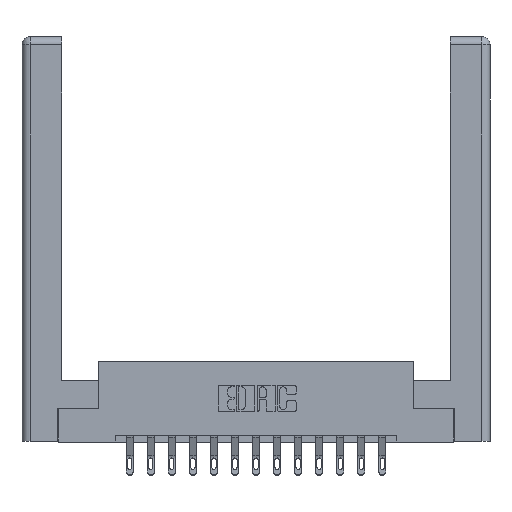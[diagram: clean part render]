
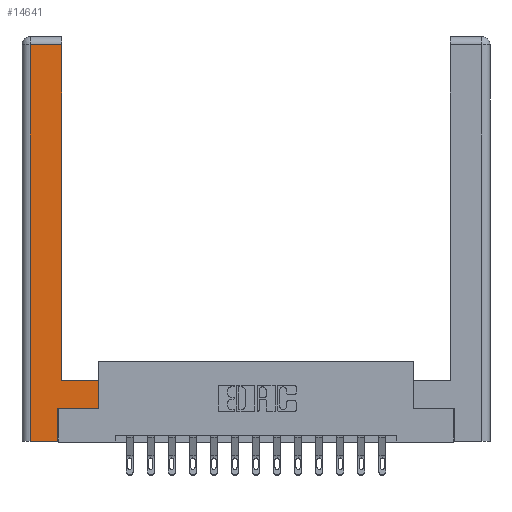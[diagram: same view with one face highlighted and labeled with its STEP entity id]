
A CAD part, top view. The second image highlights one B-rep face of the part: STEP entity #14641.
In plain terms, the highlighted planar face has unit normal (0, 0, 1).
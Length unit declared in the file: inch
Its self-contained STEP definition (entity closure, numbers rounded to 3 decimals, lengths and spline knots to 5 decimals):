
#505 = CARTESIAN_POINT ( 'NONE',  ( 0.565, 0.245, 0. ) ) ;
#565 = VECTOR ( 'NONE', #7714, 39.37008 ) ;
#623 = DIRECTION ( 'NONE',  ( -1., 0., 0. ) ) ;
#813 = VERTEX_POINT ( 'NONE', #505 ) ;
#921 = DIRECTION ( 'NONE',  ( 0., 1., 0. ) ) ;
#1195 = VERTEX_POINT ( 'NONE', #1445 ) ;
#1219 = FACE_OUTER_BOUND ( 'NONE', #9299, .T. ) ;
#1445 = CARTESIAN_POINT ( 'NONE',  ( 0.265, 0., 0. ) ) ;
#1475 = VERTEX_POINT ( 'NONE', #13911 ) ;
#1801 = CARTESIAN_POINT ( 'NONE',  ( 0.0615, 2.94, 0. ) ) ;
#1964 = CARTESIAN_POINT ( 'NONE',  ( 0.0615, 2.94, 0. ) ) ;
#2117 = CARTESIAN_POINT ( 'NONE',  ( 0.0615, 0., 0. ) ) ;
#2124 = CARTESIAN_POINT ( 'NONE',  ( 0.265, 0.245, 0. ) ) ;
#2249 = VECTOR ( 'NONE', #3115, 39.37008 ) ;
#2702 = ORIENTED_EDGE ( 'NONE', *, *, #9964, .T. ) ;
#3115 = DIRECTION ( 'NONE',  ( -1., 0., 0. ) ) ;
#3175 = EDGE_CURVE ( 'NONE', #1195, #6629, #4870, .T. ) ;
#3377 = VERTEX_POINT ( 'NONE', #10694 ) ;
#3609 = PLANE ( 'NONE',  #8350 ) ;
#3668 = LINE ( 'NONE', #12040, #7566 ) ;
#3919 = CARTESIAN_POINT ( 'NONE',  ( 0.565, 0.245, 0. ) ) ;
#4242 = DIRECTION ( 'NONE',  ( 1., 0., 0. ) ) ;
#4404 = ORIENTED_EDGE ( 'NONE', *, *, #7227, .T. ) ;
#4689 = CARTESIAN_POINT ( 'NONE',  ( 0., 0., 0. ) ) ;
#4712 = CARTESIAN_POINT ( 'NONE',  ( 0.0615, 0., 0. ) ) ;
#4793 = CARTESIAN_POINT ( 'NONE',  ( 0.295, 0.45, 0. ) ) ;
#4870 = LINE ( 'NONE', #15410, #565 ) ;
#5075 = VERTEX_POINT ( 'NONE', #1964 ) ;
#5552 = EDGE_CURVE ( 'NONE', #813, #3377, #14548, .T. ) ;
#6075 = VECTOR ( 'NONE', #12247, 39.37008 ) ;
#6571 = LINE ( 'NONE', #1801, #2249 ) ;
#6629 = VERTEX_POINT ( 'NONE', #2124 ) ;
#6631 = DIRECTION ( 'NONE',  ( 1., 0., 0. ) ) ;
#7207 = LINE ( 'NONE', #16402, #10258 ) ;
#7227 = EDGE_CURVE ( 'NONE', #6629, #813, #11699, .T. ) ;
#7566 = VECTOR ( 'NONE', #4242, 39.37008 ) ;
#7714 = DIRECTION ( 'NONE',  ( 0., 1., 0. ) ) ;
#8350 = AXIS2_PLACEMENT_3D ( 'NONE', #4689, #12789, #12743 ) ;
#8803 = ORIENTED_EDGE ( 'NONE', *, *, #13576, .T. ) ;
#9165 = EDGE_CURVE ( 'NONE', #1475, #14554, #7207, .T. ) ;
#9299 = EDGE_LOOP ( 'NONE', ( #14839, #2702, #14176, #10790, #10828, #4404, #13908, #8803 ) ) ;
#9964 = EDGE_CURVE ( 'NONE', #14554, #5075, #6571, .T. ) ;
#10258 = VECTOR ( 'NONE', #921, 39.37008 ) ;
#10264 = VECTOR ( 'NONE', #623, 39.37008 ) ;
#10490 = EDGE_CURVE ( 'NONE', #16329, #1195, #3668, .T. ) ;
#10651 = LINE ( 'NONE', #4793, #10264 ) ;
#10694 = CARTESIAN_POINT ( 'NONE',  ( 0.565, 0.45, 0. ) ) ;
#10790 = ORIENTED_EDGE ( 'NONE', *, *, #10490, .T. ) ;
#10828 = ORIENTED_EDGE ( 'NONE', *, *, #3175, .T. ) ;
#11063 = CARTESIAN_POINT ( 'NONE',  ( 0.565, 0.45, 0. ) ) ;
#11699 = LINE ( 'NONE', #3919, #16114 ) ;
#12040 = CARTESIAN_POINT ( 'NONE',  ( 0.265, 0., 0. ) ) ;
#12097 = VECTOR ( 'NONE', #16372, 39.37008 ) ;
#12247 = DIRECTION ( 'NONE',  ( 0., 1., 0. ) ) ;
#12701 = EDGE_CURVE ( 'NONE', #5075, #16329, #13475, .T. ) ;
#12743 = DIRECTION ( 'NONE',  ( -1., 0., 0. ) ) ;
#12789 = DIRECTION ( 'NONE',  ( 0., 0., -1. ) ) ;
#13475 = LINE ( 'NONE', #4712, #12097 ) ;
#13576 = EDGE_CURVE ( 'NONE', #3377, #1475, #10651, .T. ) ;
#13702 = CARTESIAN_POINT ( 'NONE',  ( 0.295, 2.94, 0. ) ) ;
#13908 = ORIENTED_EDGE ( 'NONE', *, *, #5552, .T. ) ;
#13911 = CARTESIAN_POINT ( 'NONE',  ( 0.295, 0.45, 0. ) ) ;
#14176 = ORIENTED_EDGE ( 'NONE', *, *, #12701, .T. ) ;
#14548 = LINE ( 'NONE', #11063, #6075 ) ;
#14554 = VERTEX_POINT ( 'NONE', #13702 ) ;
#14641 = ADVANCED_FACE ( 'NONE', ( #1219 ), #3609, .F. ) ;
#14839 = ORIENTED_EDGE ( 'NONE', *, *, #9165, .T. ) ;
#15410 = CARTESIAN_POINT ( 'NONE',  ( 0.265, 0.245, 0. ) ) ;
#16114 = VECTOR ( 'NONE', #6631, 39.37008 ) ;
#16329 = VERTEX_POINT ( 'NONE', #2117 ) ;
#16372 = DIRECTION ( 'NONE',  ( 0., -1., 0. ) ) ;
#16402 = CARTESIAN_POINT ( 'NONE',  ( 0.295, 3., 0. ) ) ;
